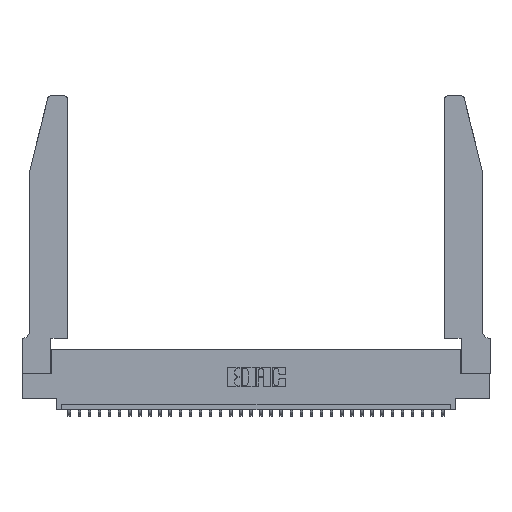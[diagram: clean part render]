
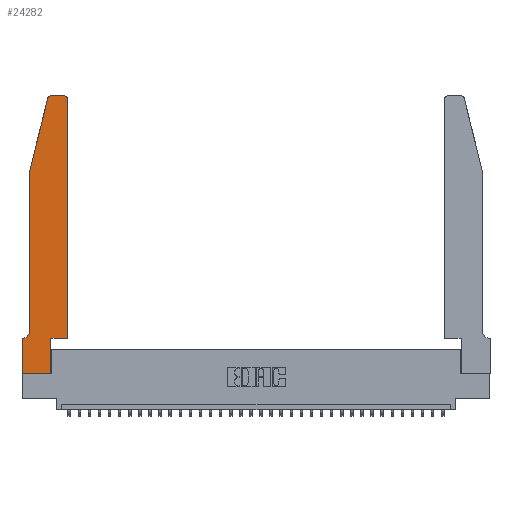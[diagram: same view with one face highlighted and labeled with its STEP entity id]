
A CAD part, top view. The second image highlights one B-rep face of the part: STEP entity #24282.
In plain terms, the highlighted planar face has unit normal (0, 0, 1).
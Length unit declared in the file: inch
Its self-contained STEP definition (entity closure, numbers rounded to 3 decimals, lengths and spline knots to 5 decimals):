
#459 = CARTESIAN_POINT ( 'NONE',  ( 0., 0.35, 0.37 ) ) ;
#721 = EDGE_CURVE ( 'NONE', #22840, #25663, #1942, .T. ) ;
#980 = ORIENTED_EDGE ( 'NONE', *, *, #8285, .T. ) ;
#1363 = CARTESIAN_POINT ( 'NONE',  ( 0.4505, 2.72, 0.37 ) ) ;
#1416 = VERTEX_POINT ( 'NONE', #17724 ) ;
#1942 = LINE ( 'NONE', #19100, #20511 ) ;
#2349 = DIRECTION ( 'NONE',  ( 0., -1., 0. ) ) ;
#2869 = VERTEX_POINT ( 'NONE', #16490 ) ;
#3018 = CIRCLE ( 'NONE', #5480, 0.07 ) ;
#3401 = LINE ( 'NONE', #5594, #22825 ) ;
#3884 = LINE ( 'NONE', #6395, #23298 ) ;
#4050 = CARTESIAN_POINT ( 'NONE',  ( 0.0055, 0.42, 0.37 ) ) ;
#5009 = EDGE_CURVE ( 'NONE', #34109, #5261, #14374, .T. ) ;
#5261 = VERTEX_POINT ( 'NONE', #7383 ) ;
#5480 = AXIS2_PLACEMENT_3D ( 'NONE', #4050, #9258, #9606 ) ;
#5575 = DIRECTION ( 'NONE',  ( 0., 0., 1. ) ) ;
#5593 = VECTOR ( 'NONE', #25619, 39.37008 ) ;
#5594 = CARTESIAN_POINT ( 'NONE',  ( 0.2865, 0.35, 0.37 ) ) ;
#6018 = VERTEX_POINT ( 'NONE', #8834 ) ;
#6331 = VECTOR ( 'NONE', #13109, 39.37008 ) ;
#6395 = CARTESIAN_POINT ( 'NONE',  ( 0.0755, 2., 0.37 ) ) ;
#6944 = VERTEX_POINT ( 'NONE', #26380 ) ;
#7041 = EDGE_CURVE ( 'NONE', #26223, #6018, #12147, .T. ) ;
#7044 = EDGE_CURVE ( 'NONE', #31260, #31762, #3018, .T. ) ;
#7116 = DIRECTION ( 'NONE',  ( 1., 0., 0. ) ) ;
#7185 = EDGE_CURVE ( 'NONE', #1416, #31260, #3884, .T. ) ;
#7383 = CARTESIAN_POINT ( 'NONE',  ( 0.4205, 2.75, 0.37 ) ) ;
#7604 = ORIENTED_EDGE ( 'NONE', *, *, #29996, .T. ) ;
#8206 = DIRECTION ( 'NONE',  ( 1., 0., 0. ) ) ;
#8285 = EDGE_CURVE ( 'NONE', #15719, #22840, #3401, .T. ) ;
#8834 = CARTESIAN_POINT ( 'NONE',  ( 0., 0., 0.37 ) ) ;
#8983 = ORIENTED_EDGE ( 'NONE', *, *, #7041, .T. ) ;
#9135 = CARTESIAN_POINT ( 'NONE',  ( 0., 0., 0.37 ) ) ;
#9144 = ORIENTED_EDGE ( 'NONE', *, *, #19177, .T. ) ;
#9258 = DIRECTION ( 'NONE',  ( 0., 0., -1. ) ) ;
#9491 = DIRECTION ( 'NONE',  ( 0., -1., 0. ) ) ;
#9606 = DIRECTION ( 'NONE',  ( -1., 0., 0. ) ) ;
#9682 = EDGE_CURVE ( 'NONE', #31762, #26223, #31525, .T. ) ;
#10122 = ORIENTED_EDGE ( 'NONE', *, *, #5009, .T. ) ;
#10598 = ORIENTED_EDGE ( 'NONE', *, *, #7185, .T. ) ;
#10643 = ORIENTED_EDGE ( 'NONE', *, *, #721, .T. ) ;
#10724 = VECTOR ( 'NONE', #29689, 39.37008 ) ;
#10743 = DIRECTION ( 'NONE',  ( 0., 0., 1. ) ) ;
#11050 = DIRECTION ( 'NONE',  ( 1., 0., 0. ) ) ;
#11549 = CARTESIAN_POINT ( 'NONE',  ( 0.0755, 2., 0.37 ) ) ;
#12147 = LINE ( 'NONE', #9135, #22459 ) ;
#12656 = LINE ( 'NONE', #33438, #5593 ) ;
#13109 = DIRECTION ( 'NONE',  ( 0., 1., 0. ) ) ;
#13404 = CARTESIAN_POINT ( 'NONE',  ( 0.0755, 0.42, 0.37 ) ) ;
#14318 = CARTESIAN_POINT ( 'NONE',  ( 0., 0., 0.37 ) ) ;
#14374 = CIRCLE ( 'NONE', #23773, 0.03 ) ;
#14815 = ORIENTED_EDGE ( 'NONE', *, *, #15034, .T. ) ;
#15034 = EDGE_CURVE ( 'NONE', #2869, #1416, #31722, .T. ) ;
#15556 = CARTESIAN_POINT ( 'NONE',  ( 0.2865, 0.35, 0.37 ) ) ;
#15719 = VERTEX_POINT ( 'NONE', #20076 ) ;
#16065 = CARTESIAN_POINT ( 'NONE',  ( 0.4205, 2.72, 0.37 ) ) ;
#16107 = EDGE_CURVE ( 'NONE', #6944, #2869, #20653, .T. ) ;
#16490 = CARTESIAN_POINT ( 'NONE',  ( 0.25487, 2.72718, 0.37 ) ) ;
#17543 = ORIENTED_EDGE ( 'NONE', *, *, #7044, .T. ) ;
#17724 = CARTESIAN_POINT ( 'NONE',  ( 0.0755, 2., 0.37 ) ) ;
#18013 = EDGE_CURVE ( 'NONE', #5261, #6944, #12656, .T. ) ;
#18505 = AXIS2_PLACEMENT_3D ( 'NONE', #20252, #28162, #7116 ) ;
#19100 = CARTESIAN_POINT ( 'NONE',  ( 0.4505, 0.35, 0.37 ) ) ;
#19177 = EDGE_CURVE ( 'NONE', #25663, #34109, #22415, .T. ) ;
#19790 = ORIENTED_EDGE ( 'NONE', *, *, #9682, .T. ) ;
#20076 = CARTESIAN_POINT ( 'NONE',  ( 0.2865, 0., 0.37 ) ) ;
#20252 = CARTESIAN_POINT ( 'NONE',  ( 0.284, 2.72, 0.37 ) ) ;
#20511 = VECTOR ( 'NONE', #11050, 39.37008 ) ;
#20653 = CIRCLE ( 'NONE', #18505, 0.03 ) ;
#20975 = DIRECTION ( 'NONE',  ( -1., 0., 0. ) ) ;
#22199 = AXIS2_PLACEMENT_3D ( 'NONE', #459, #10743, #8206 ) ;
#22415 = LINE ( 'NONE', #24025, #6331 ) ;
#22459 = VECTOR ( 'NONE', #9491, 39.37008 ) ;
#22825 = VECTOR ( 'NONE', #24277, 39.37008 ) ;
#22840 = VERTEX_POINT ( 'NONE', #15556 ) ;
#23298 = VECTOR ( 'NONE', #2349, 39.37008 ) ;
#23302 = ORIENTED_EDGE ( 'NONE', *, *, #16107, .T. ) ;
#23773 = AXIS2_PLACEMENT_3D ( 'NONE', #16065, #5575, #24036 ) ;
#24025 = CARTESIAN_POINT ( 'NONE',  ( 0.4505, 0.35, 0.37 ) ) ;
#24036 = DIRECTION ( 'NONE',  ( 1., 0., 0. ) ) ;
#24277 = DIRECTION ( 'NONE',  ( 0., 1., 0. ) ) ;
#24282 = ADVANCED_FACE ( 'NONE', ( #28745 ), #24341, .T. ) ;
#24341 = PLANE ( 'NONE',  #22199 ) ;
#24933 = VECTOR ( 'NONE', #20975, 39.37008 ) ;
#25062 = CARTESIAN_POINT ( 'NONE',  ( 0.4505, 0.35, 0.37 ) ) ;
#25619 = DIRECTION ( 'NONE',  ( -1., 0., 0. ) ) ;
#25663 = VERTEX_POINT ( 'NONE', #25062 ) ;
#25886 = ORIENTED_EDGE ( 'NONE', *, *, #18013, .T. ) ;
#26072 = VECTOR ( 'NONE', #27624, 39.37008 ) ;
#26223 = VERTEX_POINT ( 'NONE', #30511 ) ;
#26380 = CARTESIAN_POINT ( 'NONE',  ( 0.284, 2.75, 0.37 ) ) ;
#27624 = DIRECTION ( 'NONE',  ( 1., 0., 0. ) ) ;
#28162 = DIRECTION ( 'NONE',  ( 0., 0., 1. ) ) ;
#28745 = FACE_OUTER_BOUND ( 'NONE', #33541, .T. ) ;
#29689 = DIRECTION ( 'NONE',  ( -0.239, -0.971, 0. ) ) ;
#29996 = EDGE_CURVE ( 'NONE', #6018, #15719, #33453, .T. ) ;
#30511 = CARTESIAN_POINT ( 'NONE',  ( 0., 0.35, 0.37 ) ) ;
#31260 = VERTEX_POINT ( 'NONE', #13404 ) ;
#31525 = LINE ( 'NONE', #32647, #24933 ) ;
#31722 = LINE ( 'NONE', #11549, #10724 ) ;
#31762 = VERTEX_POINT ( 'NONE', #32926 ) ;
#32647 = CARTESIAN_POINT ( 'NONE',  ( 0.0755, 0.35, 0.37 ) ) ;
#32926 = CARTESIAN_POINT ( 'NONE',  ( 0.0055, 0.35, 0.37 ) ) ;
#33438 = CARTESIAN_POINT ( 'NONE',  ( 0.2605, 2.75, 0.37 ) ) ;
#33453 = LINE ( 'NONE', #14318, #26072 ) ;
#33541 = EDGE_LOOP ( 'NONE', ( #25886, #23302, #14815, #10598, #17543, #19790, #8983, #7604, #980, #10643, #9144, #10122 ) ) ;
#34109 = VERTEX_POINT ( 'NONE', #1363 ) ;
